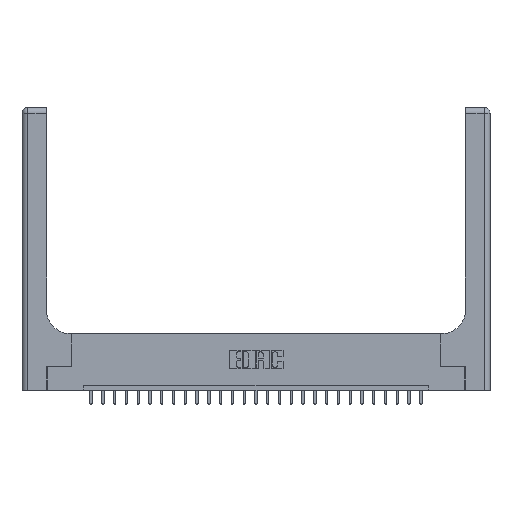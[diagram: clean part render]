
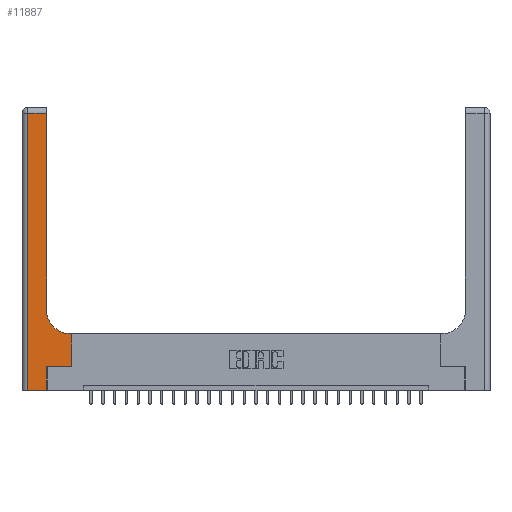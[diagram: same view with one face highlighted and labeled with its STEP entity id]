
A CAD part, top view. The second image highlights one B-rep face of the part: STEP entity #11887.
In plain terms, the highlighted planar face has unit normal (0, 0, 1).
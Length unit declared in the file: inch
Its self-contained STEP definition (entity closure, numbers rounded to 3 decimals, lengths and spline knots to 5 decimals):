
#55 = DIRECTION ( 'NONE',  ( 0., 0., -1. ) ) ;
#846 = VECTOR ( 'NONE', #4003, 39.37008 ) ;
#1424 = LINE ( 'NONE', #5783, #846 ) ;
#1522 = ORIENTED_EDGE ( 'NONE', *, *, #22888, .T. ) ;
#1830 = CARTESIAN_POINT ( 'NONE',  ( 0., 0., 0.37 ) ) ;
#2276 = DIRECTION ( 'NONE',  ( 0., 0., -1. ) ) ;
#2988 = CARTESIAN_POINT ( 'NONE',  ( 0.51, 0.6, 0.37 ) ) ;
#3045 = AXIS2_PLACEMENT_3D ( 'NONE', #11563, #2276, #6173 ) ;
#3487 = VECTOR ( 'NONE', #19440, 39.37008 ) ;
#4003 = DIRECTION ( 'NONE',  ( 0., 1., 0. ) ) ;
#4386 = VERTEX_POINT ( 'NONE', #23509 ) ;
#4489 = CARTESIAN_POINT ( 'NONE',  ( 0.06, 3., 0.37 ) ) ;
#4567 = EDGE_CURVE ( 'NONE', #6874, #18206, #9861, .T. ) ;
#4632 = VECTOR ( 'NONE', #15807, 39.37008 ) ;
#4896 = DIRECTION ( 'NONE',  ( 1., 0., 0. ) ) ;
#5139 = ORIENTED_EDGE ( 'NONE', *, *, #10712, .T. ) ;
#5273 = EDGE_LOOP ( 'NONE', ( #5139, #15821, #12136, #16631, #21399, #1522, #20515, #7047, #8771 ) ) ;
#5372 = CARTESIAN_POINT ( 'NONE',  ( 0.26, 0.6, 0.37 ) ) ;
#5783 = CARTESIAN_POINT ( 'NONE',  ( 0.265, 0., 0.37 ) ) ;
#5998 = VECTOR ( 'NONE', #4896, 39.37008 ) ;
#6035 = VECTOR ( 'NONE', #8260, 39.37008 ) ;
#6173 = DIRECTION ( 'NONE',  ( 1., 0., 0. ) ) ;
#6412 = VECTOR ( 'NONE', #19410, 39.37008 ) ;
#6563 = CARTESIAN_POINT ( 'NONE',  ( 0., 2.94, 0.37 ) ) ;
#6716 = FACE_OUTER_BOUND ( 'NONE', #5273, .T. ) ;
#6792 = VERTEX_POINT ( 'NONE', #19277 ) ;
#6804 = VERTEX_POINT ( 'NONE', #9913 ) ;
#6874 = VERTEX_POINT ( 'NONE', #12043 ) ;
#7047 = ORIENTED_EDGE ( 'NONE', *, *, #4567, .T. ) ;
#7087 = EDGE_CURVE ( 'NONE', #4386, #6792, #1424, .T. ) ;
#8183 = VERTEX_POINT ( 'NONE', #13119 ) ;
#8260 = DIRECTION ( 'NONE',  ( -1., 0., 0. ) ) ;
#8771 = ORIENTED_EDGE ( 'NONE', *, *, #19074, .T. ) ;
#8784 = CARTESIAN_POINT ( 'NONE',  ( 0.265, 0.25, 0.37 ) ) ;
#9197 = DIRECTION ( 'NONE',  ( 1., 0., 0. ) ) ;
#9430 = LINE ( 'NONE', #23164, #6412 ) ;
#9861 = LINE ( 'NONE', #5372, #11359 ) ;
#9913 = CARTESIAN_POINT ( 'NONE',  ( 0.528, 0.25, 0.37 ) ) ;
#10070 = CIRCLE ( 'NONE', #3045, 0.25 ) ;
#10155 = EDGE_CURVE ( 'NONE', #8183, #4386, #22677, .T. ) ;
#10712 = EDGE_CURVE ( 'NONE', #15544, #12421, #9430, .T. ) ;
#11359 = VECTOR ( 'NONE', #18622, 39.37008 ) ;
#11467 = EDGE_CURVE ( 'NONE', #23217, #8183, #15187, .T. ) ;
#11563 = CARTESIAN_POINT ( 'NONE',  ( 0.51, 0.85, 0.37 ) ) ;
#11780 = CARTESIAN_POINT ( 'NONE',  ( 0.06, 2.94, 0.37 ) ) ;
#11887 = ADVANCED_FACE ( 'NONE', ( #6716 ), #15526, .F. ) ;
#12043 = CARTESIAN_POINT ( 'NONE',  ( 0.528, 0.6, 0.37 ) ) ;
#12136 = ORIENTED_EDGE ( 'NONE', *, *, #11467, .T. ) ;
#12421 = VERTEX_POINT ( 'NONE', #21822 ) ;
#12952 = EDGE_CURVE ( 'NONE', #12421, #23217, #21077, .T. ) ;
#13119 = CARTESIAN_POINT ( 'NONE',  ( 0.06, 0., 0.37 ) ) ;
#13168 = LINE ( 'NONE', #21339, #3487 ) ;
#15187 = LINE ( 'NONE', #4489, #4632 ) ;
#15526 = PLANE ( 'NONE',  #16398 ) ;
#15544 = VERTEX_POINT ( 'NONE', #19573 ) ;
#15807 = DIRECTION ( 'NONE',  ( 0., -1., 0. ) ) ;
#15821 = ORIENTED_EDGE ( 'NONE', *, *, #12952, .T. ) ;
#16398 = AXIS2_PLACEMENT_3D ( 'NONE', #19142, #55, #23137 ) ;
#16631 = ORIENTED_EDGE ( 'NONE', *, *, #10155, .T. ) ;
#18206 = VERTEX_POINT ( 'NONE', #2988 ) ;
#18622 = DIRECTION ( 'NONE',  ( -1., 0., 0. ) ) ;
#19074 = EDGE_CURVE ( 'NONE', #18206, #15544, #10070, .T. ) ;
#19142 = CARTESIAN_POINT ( 'NONE',  ( 0., 3., 0.37 ) ) ;
#19277 = CARTESIAN_POINT ( 'NONE',  ( 0.265, 0.25, 0.37 ) ) ;
#19410 = DIRECTION ( 'NONE',  ( 0., 1., 0. ) ) ;
#19440 = DIRECTION ( 'NONE',  ( 0., 1., 0. ) ) ;
#19573 = CARTESIAN_POINT ( 'NONE',  ( 0.26, 0.85, 0.37 ) ) ;
#20515 = ORIENTED_EDGE ( 'NONE', *, *, #24066, .T. ) ;
#21077 = LINE ( 'NONE', #6563, #6035 ) ;
#21339 = CARTESIAN_POINT ( 'NONE',  ( 0.528, 0.25, 0.37 ) ) ;
#21399 = ORIENTED_EDGE ( 'NONE', *, *, #7087, .T. ) ;
#21822 = CARTESIAN_POINT ( 'NONE',  ( 0.26, 2.94, 0.37 ) ) ;
#22677 = LINE ( 'NONE', #1830, #24489 ) ;
#22820 = LINE ( 'NONE', #8784, #5998 ) ;
#22888 = EDGE_CURVE ( 'NONE', #6792, #6804, #22820, .T. ) ;
#23137 = DIRECTION ( 'NONE',  ( -1., 0., 0. ) ) ;
#23164 = CARTESIAN_POINT ( 'NONE',  ( 0.26, 3., 0.37 ) ) ;
#23217 = VERTEX_POINT ( 'NONE', #11780 ) ;
#23509 = CARTESIAN_POINT ( 'NONE',  ( 0.265, 0., 0.37 ) ) ;
#24066 = EDGE_CURVE ( 'NONE', #6804, #6874, #13168, .T. ) ;
#24489 = VECTOR ( 'NONE', #9197, 39.37008 ) ;
